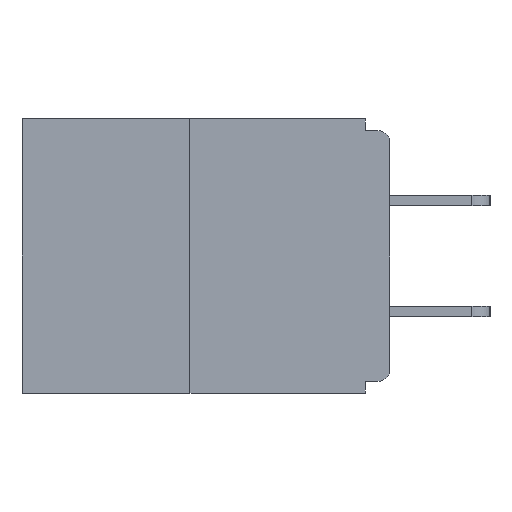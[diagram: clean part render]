
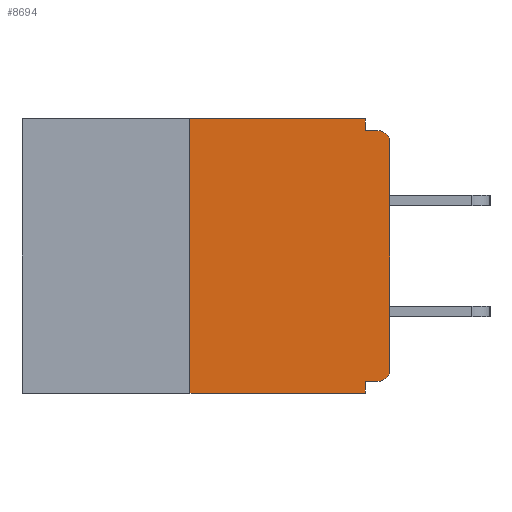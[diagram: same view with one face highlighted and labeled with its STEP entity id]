
A CAD part, left-side view. The second image highlights one B-rep face of the part: STEP entity #8694.
In plain terms, the highlighted planar face has unit normal (-1, 0, 0).
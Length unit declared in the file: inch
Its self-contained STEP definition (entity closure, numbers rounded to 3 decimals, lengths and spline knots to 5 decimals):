
#19 = DIRECTION ( 'NONE',  ( -1., 0., 0. ) ) ;
#25 = EDGE_CURVE ( 'NONE', #2776, #22972, #6612, .T. ) ;
#185 = ORIENTED_EDGE ( 'NONE', *, *, #23735, .T. ) ;
#194 = EDGE_CURVE ( 'NONE', #3195, #8375, #14890, .T. ) ;
#245 = EDGE_CURVE ( 'NONE', #20246, #5201, #2267, .T. ) ;
#316 = CARTESIAN_POINT ( 'NONE',  ( 0., 0., -0.015 ) ) ;
#371 = CARTESIAN_POINT ( 'NONE',  ( 0., 0.015, -0.03 ) ) ;
#2069 = VERTEX_POINT ( 'NONE', #9540 ) ;
#2267 = CIRCLE ( 'NONE', #21409, 0.015 ) ;
#2611 = CARTESIAN_POINT ( 'NONE',  ( 0., 0.031, -0.328 ) ) ;
#2627 = CARTESIAN_POINT ( 'NONE',  ( 0., 0., -0.328 ) ) ;
#2693 = ORIENTED_EDGE ( 'NONE', *, *, #17626, .F. ) ;
#2776 = VERTEX_POINT ( 'NONE', #4560 ) ;
#3035 = VERTEX_POINT ( 'NONE', #17639 ) ;
#3195 = VERTEX_POINT ( 'NONE', #20231 ) ;
#3254 = DIRECTION ( 'NONE',  ( 0., 0., -1. ) ) ;
#4220 = CIRCLE ( 'NONE', #19953, 0.015 ) ;
#4560 = CARTESIAN_POINT ( 'NONE',  ( 0., 0.25, -0.343 ) ) ;
#4768 = VECTOR ( 'NONE', #4979, 39.37008 ) ;
#4979 = DIRECTION ( 'NONE',  ( 0., 0., -1. ) ) ;
#5201 = VERTEX_POINT ( 'NONE', #11212 ) ;
#5660 = VECTOR ( 'NONE', #6492, 39.37008 ) ;
#6237 = EDGE_CURVE ( 'NONE', #5201, #3035, #11465, .T. ) ;
#6492 = DIRECTION ( 'NONE',  ( 0., 0., 1. ) ) ;
#6612 = LINE ( 'NONE', #18281, #5660 ) ;
#6923 = LINE ( 'NONE', #20820, #4768 ) ;
#6939 = DIRECTION ( 'NONE',  ( 1., 0., 0. ) ) ;
#7575 = VECTOR ( 'NONE', #17814, 39.37008 ) ;
#7655 = ORIENTED_EDGE ( 'NONE', *, *, #16164, .F. ) ;
#7970 = ORIENTED_EDGE ( 'NONE', *, *, #6237, .T. ) ;
#8375 = VERTEX_POINT ( 'NONE', #13938 ) ;
#8694 = ADVANCED_FACE ( 'NONE', ( #12766 ), #15221, .F. ) ;
#9066 = EDGE_CURVE ( 'NONE', #20246, #18023, #16216, .T. ) ;
#9130 = CARTESIAN_POINT ( 'NONE',  ( 0., 0.46, 0. ) ) ;
#9540 = CARTESIAN_POINT ( 'NONE',  ( 0., 0.031, -0.343 ) ) ;
#9641 = CARTESIAN_POINT ( 'NONE',  ( 0., 0., 0. ) ) ;
#9793 = DIRECTION ( 'NONE',  ( 0., -1., 0. ) ) ;
#10083 = ORIENTED_EDGE ( 'NONE', *, *, #14878, .F. ) ;
#10518 = DIRECTION ( 'NONE',  ( 0., 1., 0. ) ) ;
#11212 = CARTESIAN_POINT ( 'NONE',  ( 0., 0., -0.313 ) ) ;
#11465 = LINE ( 'NONE', #9641, #20950 ) ;
#11765 = DIRECTION ( 'NONE',  ( 0., 0., -1. ) ) ;
#11870 = AXIS2_PLACEMENT_3D ( 'NONE', #9130, #6939, #14827 ) ;
#12766 = FACE_OUTER_BOUND ( 'NONE', #21989, .T. ) ;
#12823 = ORIENTED_EDGE ( 'NONE', *, *, #9066, .F. ) ;
#13692 = CARTESIAN_POINT ( 'NONE',  ( 0., 0.015, -0.313 ) ) ;
#13790 = CARTESIAN_POINT ( 'NONE',  ( 0., 0.46, 0. ) ) ;
#13850 = DIRECTION ( 'NONE',  ( 0., 0., -1. ) ) ;
#13893 = VECTOR ( 'NONE', #3254, 39.37008 ) ;
#13938 = CARTESIAN_POINT ( 'NONE',  ( 0., 0.031, -0.015 ) ) ;
#14441 = CARTESIAN_POINT ( 'NONE',  ( 0., 0.015, -0.328 ) ) ;
#14607 = VECTOR ( 'NONE', #9793, 39.37008 ) ;
#14827 = DIRECTION ( 'NONE',  ( 0., 0., -1. ) ) ;
#14878 = EDGE_CURVE ( 'NONE', #22972, #3195, #19905, .T. ) ;
#14890 = LINE ( 'NONE', #18953, #13893 ) ;
#14982 = CARTESIAN_POINT ( 'NONE',  ( 0., 0.015, -0.015 ) ) ;
#15221 = PLANE ( 'NONE',  #11870 ) ;
#15872 = LINE ( 'NONE', #16506, #24572 ) ;
#16164 = EDGE_CURVE ( 'NONE', #8375, #23394, #23559, .T. ) ;
#16216 = LINE ( 'NONE', #2627, #20172 ) ;
#16506 = CARTESIAN_POINT ( 'NONE',  ( 0., 0.46, -0.343 ) ) ;
#16831 = CARTESIAN_POINT ( 'NONE',  ( 0., 0.25, 0. ) ) ;
#17626 = EDGE_CURVE ( 'NONE', #18023, #2069, #6923, .T. ) ;
#17639 = CARTESIAN_POINT ( 'NONE',  ( 0., 0., -0.03 ) ) ;
#17792 = DIRECTION ( 'NONE',  ( 0., 0., 1. ) ) ;
#17814 = DIRECTION ( 'NONE',  ( 0., -1., 0. ) ) ;
#18023 = VERTEX_POINT ( 'NONE', #2611 ) ;
#18281 = CARTESIAN_POINT ( 'NONE',  ( 0., 0.25, 0. ) ) ;
#18319 = ORIENTED_EDGE ( 'NONE', *, *, #245, .T. ) ;
#18953 = CARTESIAN_POINT ( 'NONE',  ( 0., 0.031, 0. ) ) ;
#19897 = ORIENTED_EDGE ( 'NONE', *, *, #25114, .T. ) ;
#19905 = LINE ( 'NONE', #13790, #7575 ) ;
#19953 = AXIS2_PLACEMENT_3D ( 'NONE', #371, #19, #13850 ) ;
#20172 = VECTOR ( 'NONE', #10518, 39.37008 ) ;
#20231 = CARTESIAN_POINT ( 'NONE',  ( 0., 0.031, 0. ) ) ;
#20246 = VERTEX_POINT ( 'NONE', #14441 ) ;
#20820 = CARTESIAN_POINT ( 'NONE',  ( 0., 0.031, -0.343 ) ) ;
#20950 = VECTOR ( 'NONE', #17792, 39.37008 ) ;
#21228 = ORIENTED_EDGE ( 'NONE', *, *, #25, .F. ) ;
#21409 = AXIS2_PLACEMENT_3D ( 'NONE', #13692, #21648, #11765 ) ;
#21648 = DIRECTION ( 'NONE',  ( -1., 0., 0. ) ) ;
#21989 = EDGE_LOOP ( 'NONE', ( #10083, #21228, #185, #2693, #12823, #18319, #7970, #19897, #7655, #25162 ) ) ;
#22645 = DIRECTION ( 'NONE',  ( 0., -1., 0. ) ) ;
#22972 = VERTEX_POINT ( 'NONE', #16831 ) ;
#23394 = VERTEX_POINT ( 'NONE', #14982 ) ;
#23559 = LINE ( 'NONE', #316, #14607 ) ;
#23735 = EDGE_CURVE ( 'NONE', #2776, #2069, #15872, .T. ) ;
#24572 = VECTOR ( 'NONE', #22645, 39.37008 ) ;
#25114 = EDGE_CURVE ( 'NONE', #3035, #23394, #4220, .T. ) ;
#25162 = ORIENTED_EDGE ( 'NONE', *, *, #194, .F. ) ;
